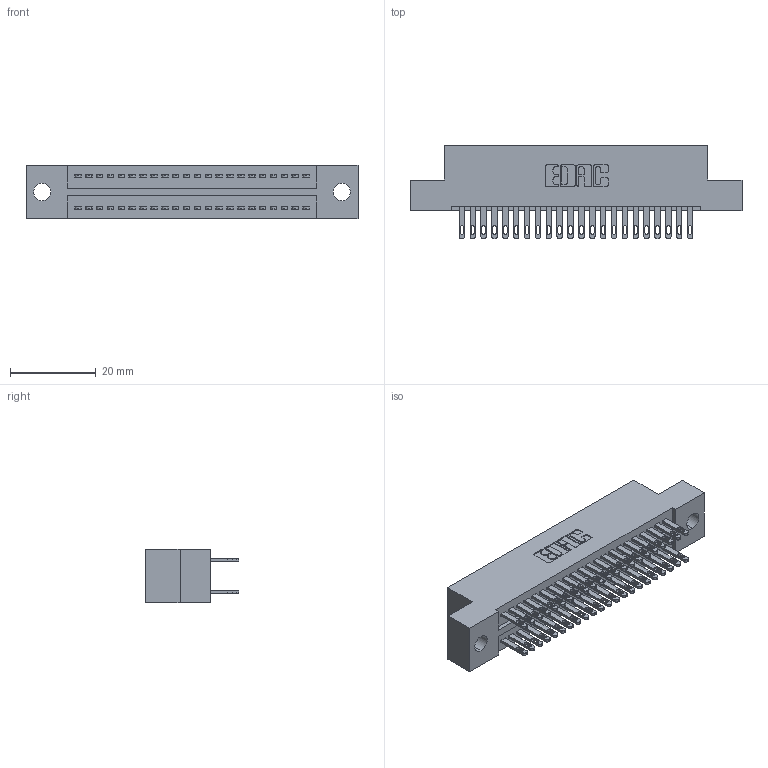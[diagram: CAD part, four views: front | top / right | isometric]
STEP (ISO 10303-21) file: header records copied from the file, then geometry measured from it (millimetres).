
FILE_DESCRIPTION (( 'STEP AP203' ), '1' );
FILE_NAME ('325-044-500-209.STEP', '2020-02-24T22:20:52', ( '' ), ( '' ), 'SwSTEP 2.0', 'SolidWorks 2016', '' );
FILE_SCHEMA (( 'CONFIG_CONTROL_DESIGN' ));
Length unit declared in the file: inch
Products named in the file (3): 325-292-001_325-293-100; 325 Part_.160 TH; 325-044-500-209
Assembly tree (45 placements, depth 2):
  325-044-500-209
    325 Part_.160 TH
    325-292-001_325-293-100  x44
Bounding box: 77.6 x 21.84 x 12.45 mm (x, y, z)
Volume: 9741.6 mm3; surface area: 11697.2 mm2
Topology: 45 solids, 45 shells, 2226 faces, 6779 edges, 4518 vertices
Faces by surface type: plane 1390, cylinder 836
Entity records: 16673 total; most frequent: CARTESIAN_POINT 2786, ORIENTED_EDGE 2722, DIRECTION 2417, EDGE_CURVE 1361, VECTOR 1229, LINE 1229, VERTEX_POINT 906, AXIS2_PLACEMENT_3D 594
